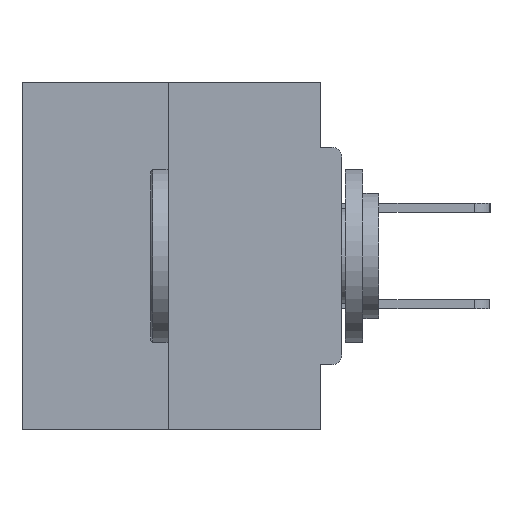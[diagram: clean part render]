
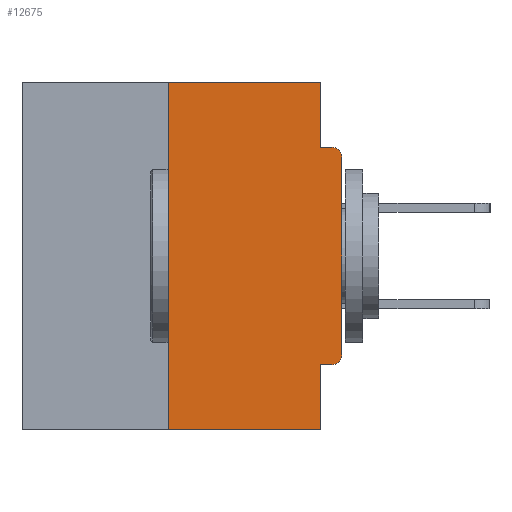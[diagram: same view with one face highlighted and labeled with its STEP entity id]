
A CAD part, left-side view. The second image highlights one B-rep face of the part: STEP entity #12675.
In plain terms, the highlighted planar face has unit normal (-1, 0, 0).
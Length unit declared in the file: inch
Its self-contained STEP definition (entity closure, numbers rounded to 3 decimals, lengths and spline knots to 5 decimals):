
#325 = PLANE ( 'NONE',  #24523 ) ;
#545 = VERTEX_POINT ( 'NONE', #21262 ) ;
#1059 = EDGE_CURVE ( 'NONE', #545, #31740, #29429, .T. ) ;
#1135 = VERTEX_POINT ( 'NONE', #8292 ) ;
#1522 = VERTEX_POINT ( 'NONE', #32589 ) ;
#1911 = FACE_OUTER_BOUND ( 'NONE', #4704, .T. ) ;
#1940 = CARTESIAN_POINT ( 'NONE',  ( 0., 0.25, 0. ) ) ;
#2049 = CIRCLE ( 'NONE', #33959, 0.015 ) ;
#2217 = LINE ( 'NONE', #3115, #30872 ) ;
#2642 = DIRECTION ( 'NONE',  ( 0., 1., 0. ) ) ;
#3021 = ORIENTED_EDGE ( 'NONE', *, *, #17455, .F. ) ;
#3115 = CARTESIAN_POINT ( 'NONE',  ( 0., 0., -0.4065 ) ) ;
#3324 = CARTESIAN_POINT ( 'NONE',  ( 0., 0.46, 0. ) ) ;
#3362 = EDGE_CURVE ( 'NONE', #6177, #1135, #23779, .T. ) ;
#3825 = VECTOR ( 'NONE', #30491, 39.37008 ) ;
#4677 = VECTOR ( 'NONE', #8699, 39.37008 ) ;
#4704 = EDGE_LOOP ( 'NONE', ( #5347, #21232, #20727, #34345, #26380, #28845, #8326, #10248, #17156, #3021 ) ) ;
#5347 = ORIENTED_EDGE ( 'NONE', *, *, #16284, .F. ) ;
#5553 = LINE ( 'NONE', #11509, #4677 ) ;
#6176 = AXIS2_PLACEMENT_3D ( 'NONE', #22374, #20020, #33229 ) ;
#6177 = VERTEX_POINT ( 'NONE', #26894 ) ;
#7361 = VERTEX_POINT ( 'NONE', #15758 ) ;
#7746 = CARTESIAN_POINT ( 'NONE',  ( 0., 0.25, -0.5 ) ) ;
#8183 = DIRECTION ( 'NONE',  ( 0., 0., -1. ) ) ;
#8292 = CARTESIAN_POINT ( 'NONE',  ( 0., 0.015, -0.0935 ) ) ;
#8326 = ORIENTED_EDGE ( 'NONE', *, *, #8350, .T. ) ;
#8350 = EDGE_CURVE ( 'NONE', #17022, #6177, #21627, .T. ) ;
#8623 = DIRECTION ( 'NONE',  ( -1., 0., 0. ) ) ;
#8699 = DIRECTION ( 'NONE',  ( 0., -1., 0. ) ) ;
#8799 = DIRECTION ( 'NONE',  ( 0., -1., 0. ) ) ;
#8807 = EDGE_CURVE ( 'NONE', #1522, #545, #2217, .T. ) ;
#9088 = DIRECTION ( 'NONE',  ( 0., 0., -1. ) ) ;
#9606 = CARTESIAN_POINT ( 'NONE',  ( 0., 0., 0. ) ) ;
#9634 = LINE ( 'NONE', #26709, #27283 ) ;
#10248 = ORIENTED_EDGE ( 'NONE', *, *, #3362, .T. ) ;
#10725 = DIRECTION ( 'NONE',  ( 1., 0., 0. ) ) ;
#10797 = EDGE_CURVE ( 'NONE', #1522, #17022, #2049, .T. ) ;
#11042 = VERTEX_POINT ( 'NONE', #1940 ) ;
#11383 = VECTOR ( 'NONE', #8183, 39.37008 ) ;
#11509 = CARTESIAN_POINT ( 'NONE',  ( 0., 0.46, -0.5 ) ) ;
#12165 = VERTEX_POINT ( 'NONE', #22841 ) ;
#12554 = VECTOR ( 'NONE', #33443, 39.37008 ) ;
#12675 = ADVANCED_FACE ( 'NONE', ( #1911 ), #325, .F. ) ;
#14077 = CARTESIAN_POINT ( 'NONE',  ( 0., 0., -0.0935 ) ) ;
#15758 = CARTESIAN_POINT ( 'NONE',  ( 0., 0.031, 0. ) ) ;
#16284 = EDGE_CURVE ( 'NONE', #11042, #7361, #28232, .T. ) ;
#17022 = VERTEX_POINT ( 'NONE', #24859 ) ;
#17156 = ORIENTED_EDGE ( 'NONE', *, *, #25863, .F. ) ;
#17455 = EDGE_CURVE ( 'NONE', #7361, #12165, #9634, .T. ) ;
#18485 = EDGE_CURVE ( 'NONE', #28016, #11042, #19705, .T. ) ;
#19289 = CARTESIAN_POINT ( 'NONE',  ( 0., 0.46, 0. ) ) ;
#19705 = LINE ( 'NONE', #33113, #12554 ) ;
#20020 = DIRECTION ( 'NONE',  ( -1., 0., 0. ) ) ;
#20727 = ORIENTED_EDGE ( 'NONE', *, *, #28170, .T. ) ;
#21232 = ORIENTED_EDGE ( 'NONE', *, *, #18485, .F. ) ;
#21262 = CARTESIAN_POINT ( 'NONE',  ( 0., 0.031, -0.4065 ) ) ;
#21393 = DIRECTION ( 'NONE',  ( 0., 0., -1. ) ) ;
#21627 = LINE ( 'NONE', #9606, #24161 ) ;
#22374 = CARTESIAN_POINT ( 'NONE',  ( 0., 0.015, -0.1085 ) ) ;
#22841 = CARTESIAN_POINT ( 'NONE',  ( 0., 0.031, -0.0935 ) ) ;
#23779 = CIRCLE ( 'NONE', #6176, 0.015 ) ;
#24043 = CARTESIAN_POINT ( 'NONE',  ( 0., 0.031, -0.5 ) ) ;
#24161 = VECTOR ( 'NONE', #30985, 39.37008 ) ;
#24523 = AXIS2_PLACEMENT_3D ( 'NONE', #19289, #10725, #21393 ) ;
#24859 = CARTESIAN_POINT ( 'NONE',  ( 0., 0., -0.3915 ) ) ;
#25135 = CARTESIAN_POINT ( 'NONE',  ( 0., 0.015, -0.3915 ) ) ;
#25863 = EDGE_CURVE ( 'NONE', #12165, #1135, #33245, .T. ) ;
#26380 = ORIENTED_EDGE ( 'NONE', *, *, #8807, .F. ) ;
#26709 = CARTESIAN_POINT ( 'NONE',  ( 0., 0.031, 0. ) ) ;
#26894 = CARTESIAN_POINT ( 'NONE',  ( 0., 0., -0.1085 ) ) ;
#27283 = VECTOR ( 'NONE', #29434, 39.37008 ) ;
#28016 = VERTEX_POINT ( 'NONE', #7746 ) ;
#28170 = EDGE_CURVE ( 'NONE', #28016, #31740, #5553, .T. ) ;
#28232 = LINE ( 'NONE', #3324, #3825 ) ;
#28845 = ORIENTED_EDGE ( 'NONE', *, *, #10797, .T. ) ;
#29429 = LINE ( 'NONE', #32274, #11383 ) ;
#29434 = DIRECTION ( 'NONE',  ( 0., 0., -1. ) ) ;
#30491 = DIRECTION ( 'NONE',  ( 0., -1., 0. ) ) ;
#30872 = VECTOR ( 'NONE', #2642, 39.37008 ) ;
#30985 = DIRECTION ( 'NONE',  ( 0., 0., 1. ) ) ;
#31740 = VERTEX_POINT ( 'NONE', #24043 ) ;
#32274 = CARTESIAN_POINT ( 'NONE',  ( 0., 0.031, -0.5 ) ) ;
#32589 = CARTESIAN_POINT ( 'NONE',  ( 0., 0.015, -0.4065 ) ) ;
#33113 = CARTESIAN_POINT ( 'NONE',  ( 0., 0.25, 0. ) ) ;
#33229 = DIRECTION ( 'NONE',  ( 0., 0., -1. ) ) ;
#33245 = LINE ( 'NONE', #14077, #34548 ) ;
#33443 = DIRECTION ( 'NONE',  ( 0., 0., 1. ) ) ;
#33959 = AXIS2_PLACEMENT_3D ( 'NONE', #25135, #8623, #9088 ) ;
#34345 = ORIENTED_EDGE ( 'NONE', *, *, #1059, .F. ) ;
#34548 = VECTOR ( 'NONE', #8799, 39.37008 ) ;
